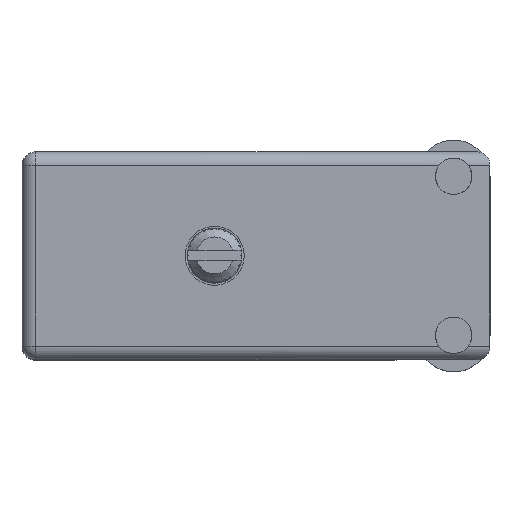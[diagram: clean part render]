
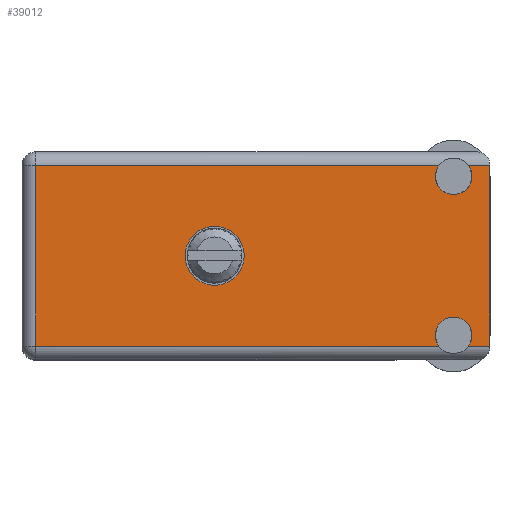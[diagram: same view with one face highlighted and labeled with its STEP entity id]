
A CAD part, top view. The second image highlights one B-rep face of the part: STEP entity #39012.
In plain terms, the highlighted face is planar.
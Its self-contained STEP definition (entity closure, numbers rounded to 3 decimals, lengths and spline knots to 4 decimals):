
#8458 = DIRECTION ( 'NONE',  ( 0., 0., 1. ) ) ;
#9459 = CARTESIAN_POINT ( 'NONE',  ( 1.484, 0.906, -0.631 ) ) ;
#12231 = VERTEX_POINT ( 'NONE', #141196 ) ;
#13109 = DIRECTION ( 'NONE',  ( 1., 0., 0. ) ) ;
#17594 = CARTESIAN_POINT ( 'NONE',  ( 1.484, 0.906, -0.084 ) ) ;
#18751 = FACE_OUTER_BOUND ( 'NONE', #61876, .T. ) ;
#20697 = PLANE ( 'NONE',  #145401 ) ;
#22784 = DIRECTION ( 'NONE',  ( 0., 1., 0. ) ) ;
#25435 = LINE ( 'NONE', #145162, #90125 ) ;
#25477 = EDGE_CURVE ( 'NONE', #75348, #12231, #124763, .T. ) ;
#28351 = CARTESIAN_POINT ( 'NONE',  ( 1.4336, 0.906, -0.668 ) ) ;
#28867 = AXIS2_PLACEMENT_3D ( 'NONE', #9459, #160338, #8458 ) ;
#30265 = DIRECTION ( 'NONE',  ( 0., 0., 1. ) ) ;
#32079 = CIRCLE ( 'NONE', #57735, 0.1015 ) ;
#33827 = CIRCLE ( 'NONE', #59472, 0.1015 ) ;
#37343 = DIRECTION ( 'NONE',  ( -1., 0., 0. ) ) ;
#38631 = CIRCLE ( 'NONE', #57837, 0.0625 ) ;
#39012 = ADVANCED_FACE ( 'NONE', ( #125333, #18751 ), #20697, .T. ) ;
#40927 = EDGE_CURVE ( 'NONE', #50399, #105071, #125199, .T. ) ;
#44288 = CARTESIAN_POINT ( 'NONE',  ( 1.5344, 0.906, -0.668 ) ) ;
#47896 = DIRECTION ( 'NONE',  ( 0., 0., 1. ) ) ;
#50399 = VERTEX_POINT ( 'NONE', #191172 ) ;
#51487 = DIRECTION ( 'NONE',  ( 0., 1., 0. ) ) ;
#52505 = VERTEX_POINT ( 'NONE', #44288 ) ;
#53409 = AXIS2_PLACEMENT_3D ( 'NONE', #96739, #51487, #53447 ) ;
#53447 = DIRECTION ( 'NONE',  ( 0., 0., 1. ) ) ;
#57399 = VERTEX_POINT ( 'NONE', #134451 ) ;
#57735 = AXIS2_PLACEMENT_3D ( 'NONE', #101149, #22784, #132350 ) ;
#57837 = AXIS2_PLACEMENT_3D ( 'NONE', #17594, #157358, #78871 ) ;
#59472 = AXIS2_PLACEMENT_3D ( 'NONE', #137049, #60579, #106822 ) ;
#60579 = DIRECTION ( 'NONE',  ( 0., 1., 0. ) ) ;
#61876 = EDGE_LOOP ( 'NONE', ( #157196, #181639, #68653, #80699, #187663, #121656, #189923, #165651, #88995, #75806 ) ) ;
#62108 = VERTEX_POINT ( 'NONE', #153875 ) ;
#64348 = VECTOR ( 'NONE', #37343, 39.3701 ) ;
#66295 = CARTESIAN_POINT ( 'NONE',  ( 1.484, 0.906, -0.1465 ) ) ;
#66772 = CARTESIAN_POINT ( 'NONE',  ( 1.609, 0.906, -0.668 ) ) ;
#68653 = ORIENTED_EDGE ( 'NONE', *, *, #194914, .F. ) ;
#75348 = VERTEX_POINT ( 'NONE', #66772 ) ;
#75806 = ORIENTED_EDGE ( 'NONE', *, *, #40927, .T. ) ;
#76014 = CARTESIAN_POINT ( 'NONE',  ( 0.047, 0.906, -0.047 ) ) ;
#78871 = DIRECTION ( 'NONE',  ( 0., 0., 1. ) ) ;
#80699 = ORIENTED_EDGE ( 'NONE', *, *, #126515, .T. ) ;
#81985 = DIRECTION ( 'NONE',  ( 0., 1., 0. ) ) ;
#88995 = ORIENTED_EDGE ( 'NONE', *, *, #89286, .T. ) ;
#89286 = EDGE_CURVE ( 'NONE', #153978, #50399, #25435, .T. ) ;
#90125 = VECTOR ( 'NONE', #189472, 39.3701 ) ;
#91046 = VERTEX_POINT ( 'NONE', #66295 ) ;
#92987 = DIRECTION ( 'NONE',  ( 0., 0., 1. ) ) ;
#94906 = CARTESIAN_POINT ( 'NONE',  ( 0.6625, 0.906, -0.459 ) ) ;
#96739 = CARTESIAN_POINT ( 'NONE',  ( 1.484, 0.906, -0.631 ) ) ;
#97983 = VERTEX_POINT ( 'NONE', #94906 ) ;
#99986 = EDGE_CURVE ( 'NONE', #147124, #97983, #33827, .T. ) ;
#101149 = CARTESIAN_POINT ( 'NONE',  ( 0.6625, 0.906, -0.3575 ) ) ;
#102205 = EDGE_CURVE ( 'NONE', #105071, #62108, #185034, .T. ) ;
#103178 = EDGE_CURVE ( 'NONE', #91046, #62108, #194509, .T. ) ;
#105071 = VERTEX_POINT ( 'NONE', #76014 ) ;
#105074 = CARTESIAN_POINT ( 'NONE',  ( 1.484, 0.906, -0.5685 ) ) ;
#106822 = DIRECTION ( 'NONE',  ( 0., 0., 1. ) ) ;
#115582 = CIRCLE ( 'NONE', #28867, 0.0625 ) ;
#121656 = ORIENTED_EDGE ( 'NONE', *, *, #195470, .T. ) ;
#123428 = DIRECTION ( 'NONE',  ( 1., 0., 0. ) ) ;
#123445 = EDGE_CURVE ( 'NONE', #97983, #147124, #32079, .T. ) ;
#124763 = LINE ( 'NONE', #137857, #131666 ) ;
#125199 = LINE ( 'NONE', #186590, #126429 ) ;
#125333 = FACE_BOUND ( 'NONE', #134480, .T. ) ;
#126429 = VECTOR ( 'NONE', #184582, 39.3701 ) ;
#126515 = EDGE_CURVE ( 'NONE', #57399, #12231, #137551, .T. ) ;
#131653 = EDGE_CURVE ( 'NONE', #163968, #52505, #115582, .T. ) ;
#131666 = VECTOR ( 'NONE', #30265, 39.3701 ) ;
#132350 = DIRECTION ( 'NONE',  ( 0., 0., 1. ) ) ;
#132824 = CARTESIAN_POINT ( 'NONE',  ( 0., 0.906, -0.668 ) ) ;
#134451 = CARTESIAN_POINT ( 'NONE',  ( 1.5344, 0.906, -0.047 ) ) ;
#134480 = EDGE_LOOP ( 'NONE', ( #166684, #179283 ) ) ;
#136559 = CARTESIAN_POINT ( 'NONE',  ( 1.609, 0.906, -0.047 ) ) ;
#136748 = CARTESIAN_POINT ( 'NONE',  ( 1.609, 0.906, -0.047 ) ) ;
#137049 = CARTESIAN_POINT ( 'NONE',  ( 0.6625, 0.906, -0.3575 ) ) ;
#137283 = CARTESIAN_POINT ( 'NONE',  ( 1.484, 0.906, -0.084 ) ) ;
#137551 = LINE ( 'NONE', #136559, #147926 ) ;
#137857 = CARTESIAN_POINT ( 'NONE',  ( 1.609, 0.906, 0. ) ) ;
#139418 = CARTESIAN_POINT ( 'NONE',  ( 0., 0.906, -0.715 ) ) ;
#140174 = CIRCLE ( 'NONE', #53409, 0.0625 ) ;
#141196 = CARTESIAN_POINT ( 'NONE',  ( 1.609, 0.906, -0.047 ) ) ;
#145162 = CARTESIAN_POINT ( 'NONE',  ( 0., 0.906, -0.668 ) ) ;
#145401 = AXIS2_PLACEMENT_3D ( 'NONE', #139418, #81985, #47896 ) ;
#147124 = VERTEX_POINT ( 'NONE', #172146 ) ;
#147926 = VECTOR ( 'NONE', #123428, 39.3701 ) ;
#153875 = CARTESIAN_POINT ( 'NONE',  ( 1.4336, 0.906, -0.047 ) ) ;
#153978 = VERTEX_POINT ( 'NONE', #28351 ) ;
#157196 = ORIENTED_EDGE ( 'NONE', *, *, #102205, .T. ) ;
#157358 = DIRECTION ( 'NONE',  ( 0., 1., 0. ) ) ;
#160338 = DIRECTION ( 'NONE',  ( 0., 1., 0. ) ) ;
#163968 = VERTEX_POINT ( 'NONE', #105074 ) ;
#164038 = LINE ( 'NONE', #132824, #64348 ) ;
#165616 = AXIS2_PLACEMENT_3D ( 'NONE', #137283, #184581, #92987 ) ;
#165651 = ORIENTED_EDGE ( 'NONE', *, *, #170037, .F. ) ;
#166684 = ORIENTED_EDGE ( 'NONE', *, *, #99986, .F. ) ;
#170037 = EDGE_CURVE ( 'NONE', #153978, #163968, #140174, .T. ) ;
#172146 = CARTESIAN_POINT ( 'NONE',  ( 0.6625, 0.906, -0.256 ) ) ;
#179283 = ORIENTED_EDGE ( 'NONE', *, *, #123445, .F. ) ;
#181639 = ORIENTED_EDGE ( 'NONE', *, *, #103178, .F. ) ;
#184581 = DIRECTION ( 'NONE',  ( 0., 1., 0. ) ) ;
#184582 = DIRECTION ( 'NONE',  ( 0., 0., 1. ) ) ;
#184877 = VECTOR ( 'NONE', #13109, 39.3701 ) ;
#185034 = LINE ( 'NONE', #136748, #184877 ) ;
#186590 = CARTESIAN_POINT ( 'NONE',  ( 0.047, 0.906, -0.715 ) ) ;
#187663 = ORIENTED_EDGE ( 'NONE', *, *, #25477, .F. ) ;
#189472 = DIRECTION ( 'NONE',  ( -1., 0., 0. ) ) ;
#189923 = ORIENTED_EDGE ( 'NONE', *, *, #131653, .F. ) ;
#191172 = CARTESIAN_POINT ( 'NONE',  ( 0.047, 0.906, -0.668 ) ) ;
#194509 = CIRCLE ( 'NONE', #165616, 0.0625 ) ;
#194914 = EDGE_CURVE ( 'NONE', #57399, #91046, #38631, .T. ) ;
#195470 = EDGE_CURVE ( 'NONE', #75348, #52505, #164038, .T. ) ;
